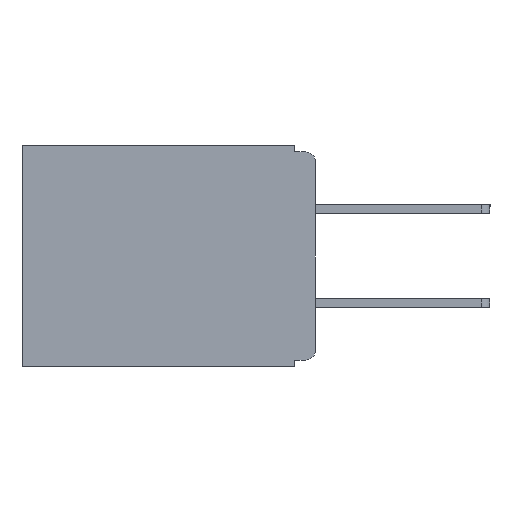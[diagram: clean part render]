
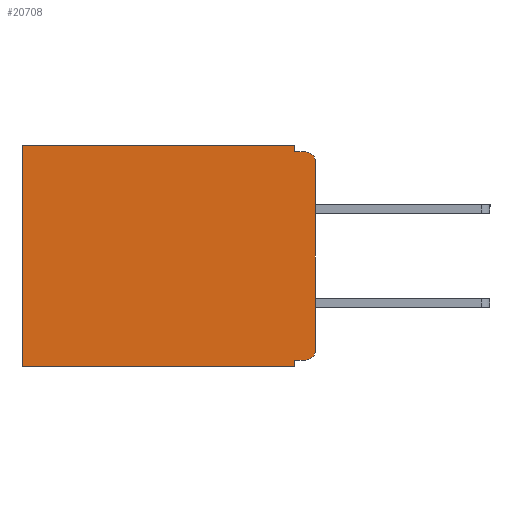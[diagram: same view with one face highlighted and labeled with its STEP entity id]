
A CAD part, left-side view. The second image highlights one B-rep face of the part: STEP entity #20708.
In plain terms, the highlighted planar face has unit normal (-1, 0, 0).
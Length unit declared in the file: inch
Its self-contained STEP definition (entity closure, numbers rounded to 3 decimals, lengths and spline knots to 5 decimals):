
#45 = ORIENTED_EDGE ( 'NONE', *, *, #18694, .T. ) ;
#75 = VECTOR ( 'NONE', #1721, 39.37008 ) ;
#119 = ORIENTED_EDGE ( 'NONE', *, *, #19259, .T. ) ;
#536 = LINE ( 'NONE', #15650, #20362 ) ;
#939 = VECTOR ( 'NONE', #6873, 39.37008 ) ;
#1155 = ORIENTED_EDGE ( 'NONE', *, *, #10878, .F. ) ;
#1234 = ORIENTED_EDGE ( 'NONE', *, *, #7352, .F. ) ;
#1575 = VECTOR ( 'NONE', #12724, 39.37008 ) ;
#1721 = DIRECTION ( 'NONE',  ( 0., 0., -1. ) ) ;
#2045 = LINE ( 'NONE', #8811, #16766 ) ;
#2140 = ORIENTED_EDGE ( 'NONE', *, *, #2198, .T. ) ;
#2198 = EDGE_CURVE ( 'NONE', #11781, #18570, #15177, .T. ) ;
#2968 = VERTEX_POINT ( 'NONE', #18663 ) ;
#3155 = EDGE_CURVE ( 'NONE', #16079, #16266, #5480, .T. ) ;
#3210 = AXIS2_PLACEMENT_3D ( 'NONE', #4284, #17716, #6217 ) ;
#3672 = VECTOR ( 'NONE', #16339, 39.37008 ) ;
#3796 = VERTEX_POINT ( 'NONE', #14129 ) ;
#4284 = CARTESIAN_POINT ( 'NONE',  ( 0.3, 0., -0.33 ) ) ;
#4439 = EDGE_CURVE ( 'NONE', #3796, #13789, #7614, .T. ) ;
#4567 = CARTESIAN_POINT ( 'NONE',  ( 0.3, 0.437, 0. ) ) ;
#4663 = LINE ( 'NONE', #7611, #75 ) ;
#4769 = EDGE_CURVE ( 'NONE', #15623, #16478, #20171, .T. ) ;
#5230 = DIRECTION ( 'NONE',  ( 0., 0., -1. ) ) ;
#5480 = LINE ( 'NONE', #13900, #939 ) ;
#5502 = CARTESIAN_POINT ( 'NONE',  ( 0.3, 0.031, 0. ) ) ;
#5658 = EDGE_LOOP ( 'NONE', ( #11464, #18358, #23889, #18978, #119, #45, #1155, #9244, #1234, #2140 ) ) ;
#5849 = CARTESIAN_POINT ( 'NONE',  ( 0.3, 0.015, -0.32 ) ) ;
#6217 = DIRECTION ( 'NONE',  ( 0., 0., -1. ) ) ;
#6873 = DIRECTION ( 'NONE',  ( 0., 0., -1. ) ) ;
#6983 = CARTESIAN_POINT ( 'NONE',  ( 0.3, 0.437, -0.33 ) ) ;
#7352 = EDGE_CURVE ( 'NONE', #11781, #16079, #2045, .T. ) ;
#7561 = LINE ( 'NONE', #9057, #18369 ) ;
#7611 = CARTESIAN_POINT ( 'NONE',  ( 0.3, 0., -0.33 ) ) ;
#7614 = LINE ( 'NONE', #5502, #22770 ) ;
#7797 = CARTESIAN_POINT ( 'NONE',  ( 0.3, 0.015, -0.305 ) ) ;
#8811 = CARTESIAN_POINT ( 'NONE',  ( 0.3, 0., -0.32 ) ) ;
#9057 = CARTESIAN_POINT ( 'NONE',  ( 0.3, 0., -0.33 ) ) ;
#9244 = ORIENTED_EDGE ( 'NONE', *, *, #3155, .F. ) ;
#9676 = CARTESIAN_POINT ( 'NONE',  ( 0.3, 0.031, -0.33 ) ) ;
#9977 = VERTEX_POINT ( 'NONE', #4567 ) ;
#10825 = DIRECTION ( 'NONE',  ( 0., 1., 0. ) ) ;
#10878 = EDGE_CURVE ( 'NONE', #16266, #2968, #7561, .T. ) ;
#10927 = DIRECTION ( 'NONE',  ( 0., 0., -1. ) ) ;
#11041 = CARTESIAN_POINT ( 'NONE',  ( 0.3, 0.031, -0.32 ) ) ;
#11464 = ORIENTED_EDGE ( 'NONE', *, *, #17642, .F. ) ;
#11781 = VERTEX_POINT ( 'NONE', #5849 ) ;
#12532 = CARTESIAN_POINT ( 'NONE',  ( 0.3, 0., 0. ) ) ;
#12537 = EDGE_CURVE ( 'NONE', #13789, #16478, #536, .T. ) ;
#12724 = DIRECTION ( 'NONE',  ( 0., 0., -1. ) ) ;
#13789 = VERTEX_POINT ( 'NONE', #23319 ) ;
#13900 = CARTESIAN_POINT ( 'NONE',  ( 0.3, 0.031, -0.33 ) ) ;
#14129 = CARTESIAN_POINT ( 'NONE',  ( 0.3, 0.031, 0. ) ) ;
#14220 = AXIS2_PLACEMENT_3D ( 'NONE', #7797, #19925, #10927 ) ;
#15177 = CIRCLE ( 'NONE', #14220, 0.015 ) ;
#15182 = CARTESIAN_POINT ( 'NONE',  ( 0.3, 0., -0.025 ) ) ;
#15623 = VERTEX_POINT ( 'NONE', #15182 ) ;
#15650 = CARTESIAN_POINT ( 'NONE',  ( 0.3, 0., -0.01 ) ) ;
#15788 = PLANE ( 'NONE',  #3210 ) ;
#15960 = CARTESIAN_POINT ( 'NONE',  ( 0.3, 0.015, -0.01 ) ) ;
#16079 = VERTEX_POINT ( 'NONE', #11041 ) ;
#16266 = VERTEX_POINT ( 'NONE', #9676 ) ;
#16339 = DIRECTION ( 'NONE',  ( 0., 1., 0. ) ) ;
#16478 = VERTEX_POINT ( 'NONE', #15960 ) ;
#16766 = VECTOR ( 'NONE', #10825, 39.37008 ) ;
#16919 = LINE ( 'NONE', #6983, #1575 ) ;
#17642 = EDGE_CURVE ( 'NONE', #15623, #18570, #4663, .T. ) ;
#17716 = DIRECTION ( 'NONE',  ( 1., 0., 0. ) ) ;
#18358 = ORIENTED_EDGE ( 'NONE', *, *, #4769, .T. ) ;
#18369 = VECTOR ( 'NONE', #24190, 39.37008 ) ;
#18570 = VERTEX_POINT ( 'NONE', #19870 ) ;
#18618 = FACE_OUTER_BOUND ( 'NONE', #5658, .T. ) ;
#18663 = CARTESIAN_POINT ( 'NONE',  ( 0.3, 0.437, -0.33 ) ) ;
#18694 = EDGE_CURVE ( 'NONE', #9977, #2968, #16919, .T. ) ;
#18978 = ORIENTED_EDGE ( 'NONE', *, *, #4439, .F. ) ;
#19259 = EDGE_CURVE ( 'NONE', #3796, #9977, #23897, .T. ) ;
#19870 = CARTESIAN_POINT ( 'NONE',  ( 0.3, 0., -0.305 ) ) ;
#19925 = DIRECTION ( 'NONE',  ( -1., 0., 0. ) ) ;
#20171 = CIRCLE ( 'NONE', #22580, 0.015 ) ;
#20362 = VECTOR ( 'NONE', #21341, 39.37008 ) ;
#20708 = ADVANCED_FACE ( 'NONE', ( #18618 ), #15788, .F. ) ;
#21341 = DIRECTION ( 'NONE',  ( 0., -1., 0. ) ) ;
#21553 = DIRECTION ( 'NONE',  ( 0., 0., -1. ) ) ;
#21574 = DIRECTION ( 'NONE',  ( -1., 0., 0. ) ) ;
#21600 = CARTESIAN_POINT ( 'NONE',  ( 0.3, 0.015, -0.025 ) ) ;
#22580 = AXIS2_PLACEMENT_3D ( 'NONE', #21600, #21574, #21553 ) ;
#22770 = VECTOR ( 'NONE', #5230, 39.37008 ) ;
#23319 = CARTESIAN_POINT ( 'NONE',  ( 0.3, 0.031, -0.01 ) ) ;
#23889 = ORIENTED_EDGE ( 'NONE', *, *, #12537, .F. ) ;
#23897 = LINE ( 'NONE', #12532, #3672 ) ;
#24190 = DIRECTION ( 'NONE',  ( 0., 1., 0. ) ) ;
